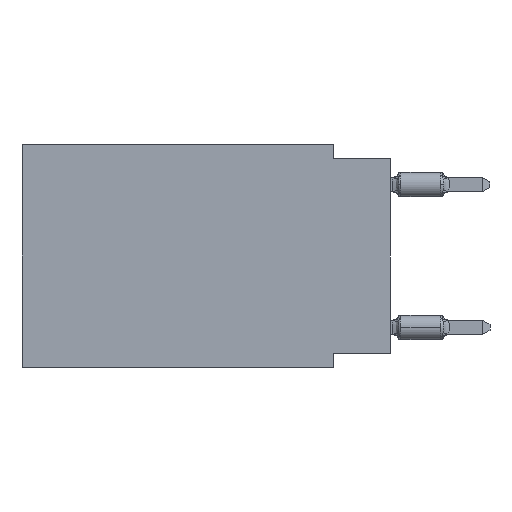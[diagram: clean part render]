
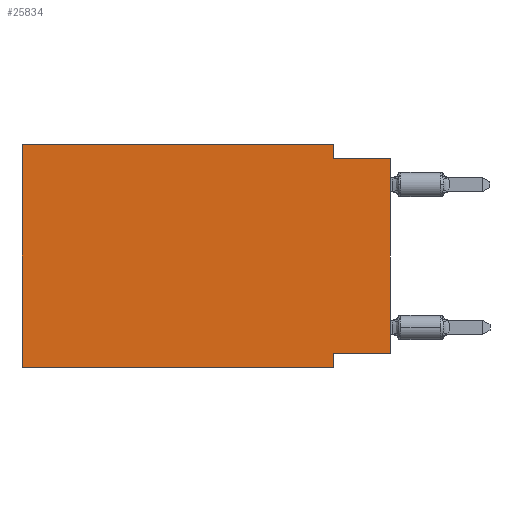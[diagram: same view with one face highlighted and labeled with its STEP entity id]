
A CAD part, left-side view. The second image highlights one B-rep face of the part: STEP entity #25834.
In plain terms, the highlighted planar face has unit normal (-1, 0, 0).
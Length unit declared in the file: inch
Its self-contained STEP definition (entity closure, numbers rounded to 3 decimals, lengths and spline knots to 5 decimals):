
#725 = VECTOR ( 'NONE', #8781, 39.37008 ) ;
#1170 = LINE ( 'NONE', #26790, #2486 ) ;
#2486 = VECTOR ( 'NONE', #35229, 39.37008 ) ;
#3093 = CARTESIAN_POINT ( 'NONE',  ( 0., 0.1, -0.365 ) ) ;
#3632 = VECTOR ( 'NONE', #35672, 39.37008 ) ;
#4356 = DIRECTION ( 'NONE',  ( 0., 0., 1. ) ) ;
#4374 = LINE ( 'NONE', #12988, #31990 ) ;
#5661 = DIRECTION ( 'NONE',  ( 1., 0., 0. ) ) ;
#6015 = VERTEX_POINT ( 'NONE', #22359 ) ;
#6990 = VERTEX_POINT ( 'NONE', #17041 ) ;
#7518 = EDGE_CURVE ( 'NONE', #12787, #32548, #15137, .T. ) ;
#7957 = VECTOR ( 'NONE', #31278, 39.37008 ) ;
#8656 = FACE_OUTER_BOUND ( 'NONE', #24054, .T. ) ;
#8713 = EDGE_CURVE ( 'NONE', #6015, #31244, #28561, .T. ) ;
#8781 = DIRECTION ( 'NONE',  ( 0., 1., 0. ) ) ;
#8849 = CARTESIAN_POINT ( 'NONE',  ( 0., 0.1, -0.39 ) ) ;
#8952 = LINE ( 'NONE', #34394, #725 ) ;
#10702 = VECTOR ( 'NONE', #4356, 39.37008 ) ;
#11104 = CARTESIAN_POINT ( 'NONE',  ( 0., 0.645, 0. ) ) ;
#12787 = VERTEX_POINT ( 'NONE', #36247 ) ;
#12988 = CARTESIAN_POINT ( 'NONE',  ( 0., 0.645, 0. ) ) ;
#13740 = CARTESIAN_POINT ( 'NONE',  ( 0., 0., -0.365 ) ) ;
#15052 = ORIENTED_EDGE ( 'NONE', *, *, #18007, .T. ) ;
#15137 = LINE ( 'NONE', #18310, #3632 ) ;
#15967 = LINE ( 'NONE', #32795, #10702 ) ;
#16435 = VERTEX_POINT ( 'NONE', #13740 ) ;
#17041 = CARTESIAN_POINT ( 'NONE',  ( 0., 0.1, -0.39 ) ) ;
#17062 = DIRECTION ( 'NONE',  ( 0., 0., -1. ) ) ;
#17443 = LINE ( 'NONE', #8849, #25694 ) ;
#18007 = EDGE_CURVE ( 'NONE', #16435, #23810, #15967, .T. ) ;
#18050 = VECTOR ( 'NONE', #31923, 39.37008 ) ;
#18310 = CARTESIAN_POINT ( 'NONE',  ( 0., 0.645, 0. ) ) ;
#18667 = CARTESIAN_POINT ( 'NONE',  ( 0., 0., -0.025 ) ) ;
#18889 = ORIENTED_EDGE ( 'NONE', *, *, #23538, .F. ) ;
#19069 = ORIENTED_EDGE ( 'NONE', *, *, #7518, .F. ) ;
#19562 = EDGE_CURVE ( 'NONE', #23856, #6990, #17443, .T. ) ;
#19883 = CARTESIAN_POINT ( 'NONE',  ( 0., 0.645, -0.39 ) ) ;
#20240 = DIRECTION ( 'NONE',  ( 0., 0., -1. ) ) ;
#21588 = ORIENTED_EDGE ( 'NONE', *, *, #35288, .F. ) ;
#22308 = ORIENTED_EDGE ( 'NONE', *, *, #32575, .T. ) ;
#22359 = CARTESIAN_POINT ( 'NONE',  ( 0., 0.1, 0. ) ) ;
#22746 = EDGE_CURVE ( 'NONE', #31244, #23810, #1170, .T. ) ;
#23298 = ORIENTED_EDGE ( 'NONE', *, *, #8713, .F. ) ;
#23392 = PLANE ( 'NONE',  #27124 ) ;
#23538 = EDGE_CURVE ( 'NONE', #16435, #23856, #8952, .T. ) ;
#23810 = VERTEX_POINT ( 'NONE', #18667 ) ;
#23847 = DIRECTION ( 'NONE',  ( 0., -1., 0. ) ) ;
#23856 = VERTEX_POINT ( 'NONE', #3093 ) ;
#24054 = EDGE_LOOP ( 'NONE', ( #15052, #24132, #23298, #21588, #19069, #22308, #34160, #18889 ) ) ;
#24132 = ORIENTED_EDGE ( 'NONE', *, *, #22746, .F. ) ;
#25694 = VECTOR ( 'NONE', #20240, 39.37008 ) ;
#25834 = ADVANCED_FACE ( 'NONE', ( #8656 ), #23392, .F. ) ;
#26790 = CARTESIAN_POINT ( 'NONE',  ( 0., 0., -0.025 ) ) ;
#27124 = AXIS2_PLACEMENT_3D ( 'NONE', #31456, #5661, #17062 ) ;
#28561 = LINE ( 'NONE', #36983, #18050 ) ;
#28647 = LINE ( 'NONE', #19883, #7957 ) ;
#31244 = VERTEX_POINT ( 'NONE', #34567 ) ;
#31278 = DIRECTION ( 'NONE',  ( 0., -1., 0. ) ) ;
#31456 = CARTESIAN_POINT ( 'NONE',  ( 0., 0.645, 0. ) ) ;
#31923 = DIRECTION ( 'NONE',  ( 0., 0., -1. ) ) ;
#31990 = VECTOR ( 'NONE', #23847, 39.37008 ) ;
#32548 = VERTEX_POINT ( 'NONE', #11104 ) ;
#32575 = EDGE_CURVE ( 'NONE', #12787, #6990, #28647, .T. ) ;
#32795 = CARTESIAN_POINT ( 'NONE',  ( 0., 0., 0. ) ) ;
#34160 = ORIENTED_EDGE ( 'NONE', *, *, #19562, .F. ) ;
#34394 = CARTESIAN_POINT ( 'NONE',  ( 0., 0., -0.365 ) ) ;
#34567 = CARTESIAN_POINT ( 'NONE',  ( 0., 0.1, -0.025 ) ) ;
#35229 = DIRECTION ( 'NONE',  ( 0., -1., 0. ) ) ;
#35288 = EDGE_CURVE ( 'NONE', #32548, #6015, #4374, .T. ) ;
#35672 = DIRECTION ( 'NONE',  ( 0., 0., 1. ) ) ;
#36247 = CARTESIAN_POINT ( 'NONE',  ( 0., 0.645, -0.39 ) ) ;
#36983 = CARTESIAN_POINT ( 'NONE',  ( 0., 0.1, 0. ) ) ;
